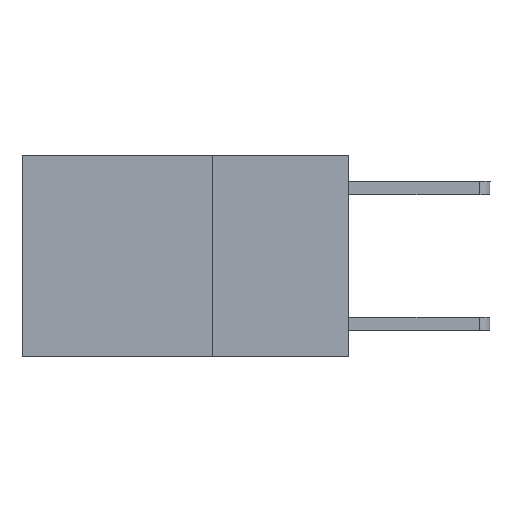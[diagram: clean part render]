
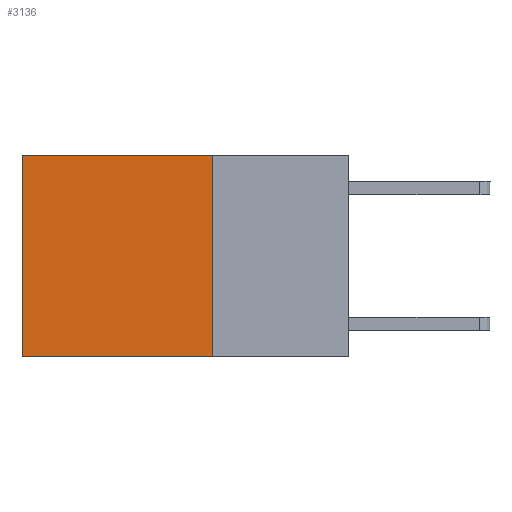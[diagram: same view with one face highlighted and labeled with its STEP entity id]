
A CAD part, left-side view. The second image highlights one B-rep face of the part: STEP entity #3136.
In plain terms, the highlighted planar face has unit normal (-1, 0, 0).
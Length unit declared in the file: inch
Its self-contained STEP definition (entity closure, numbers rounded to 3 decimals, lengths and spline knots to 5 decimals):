
#196 = ORIENTED_EDGE ( 'NONE', *, *, #4005, .T. ) ;
#327 = VECTOR ( 'NONE', #5083, 39.37008 ) ;
#432 = LINE ( 'NONE', #1813, #5270 ) ;
#519 = CARTESIAN_POINT ( 'NONE',  ( 0.2625, 0.6, -0.37 ) ) ;
#741 = FACE_OUTER_BOUND ( 'NONE', #8621, .T. ) ;
#1162 = VERTEX_POINT ( 'NONE', #1245 ) ;
#1245 = CARTESIAN_POINT ( 'NONE',  ( 0.2625, 0.25, 0. ) ) ;
#1481 = DIRECTION ( 'NONE',  ( 0., 0., -1. ) ) ;
#1813 = CARTESIAN_POINT ( 'NONE',  ( 0.2625, 0.25, 0. ) ) ;
#1900 = AXIS2_PLACEMENT_3D ( 'NONE', #6585, #5935, #8814 ) ;
#1911 = VECTOR ( 'NONE', #1481, 39.37008 ) ;
#2481 = VERTEX_POINT ( 'NONE', #519 ) ;
#2622 = EDGE_CURVE ( 'NONE', #1162, #2864, #8687, .T. ) ;
#2756 = ORIENTED_EDGE ( 'NONE', *, *, #6959, .F. ) ;
#2864 = VERTEX_POINT ( 'NONE', #3646 ) ;
#2927 = CARTESIAN_POINT ( 'NONE',  ( 0.2625, 0.6, 0. ) ) ;
#3009 = PLANE ( 'NONE',  #1900 ) ;
#3086 = LINE ( 'NONE', #8050, #6193 ) ;
#3136 = ADVANCED_FACE ( 'NONE', ( #741 ), #3009, .F. ) ;
#3646 = CARTESIAN_POINT ( 'NONE',  ( 0.2625, 0.6, 0. ) ) ;
#4005 = EDGE_CURVE ( 'NONE', #2864, #2481, #8578, .T. ) ;
#4430 = DIRECTION ( 'NONE',  ( 0., 1., 0. ) ) ;
#4987 = VERTEX_POINT ( 'NONE', #6584 ) ;
#5083 = DIRECTION ( 'NONE',  ( 0., 1., 0. ) ) ;
#5270 = VECTOR ( 'NONE', #8414, 39.37008 ) ;
#5402 = EDGE_CURVE ( 'NONE', #4987, #2481, #3086, .T. ) ;
#5935 = DIRECTION ( 'NONE',  ( 1., 0., 0. ) ) ;
#6164 = ORIENTED_EDGE ( 'NONE', *, *, #5402, .F. ) ;
#6193 = VECTOR ( 'NONE', #4430, 39.37008 ) ;
#6584 = CARTESIAN_POINT ( 'NONE',  ( 0.2625, 0.25, -0.37 ) ) ;
#6585 = CARTESIAN_POINT ( 'NONE',  ( 0.2625, 0.25, 0. ) ) ;
#6959 = EDGE_CURVE ( 'NONE', #1162, #4987, #432, .T. ) ;
#7054 = ORIENTED_EDGE ( 'NONE', *, *, #2622, .T. ) ;
#8050 = CARTESIAN_POINT ( 'NONE',  ( 0.2625, 0.25, -0.37 ) ) ;
#8414 = DIRECTION ( 'NONE',  ( 0., 0., -1. ) ) ;
#8578 = LINE ( 'NONE', #2927, #1911 ) ;
#8621 = EDGE_LOOP ( 'NONE', ( #196, #6164, #2756, #7054 ) ) ;
#8687 = LINE ( 'NONE', #8784, #327 ) ;
#8784 = CARTESIAN_POINT ( 'NONE',  ( 0.2625, 0.25, 0. ) ) ;
#8814 = DIRECTION ( 'NONE',  ( 0., 0., -1. ) ) ;
